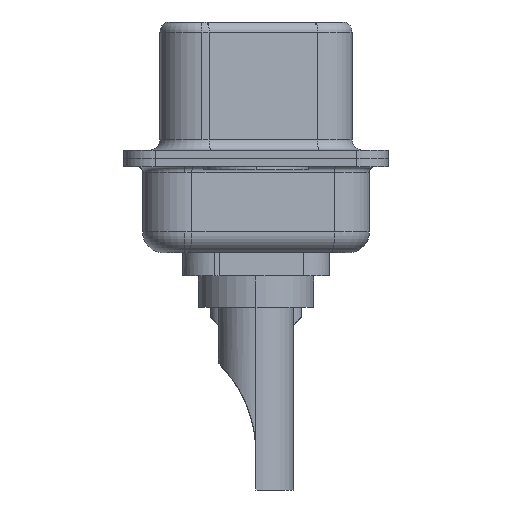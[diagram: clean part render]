
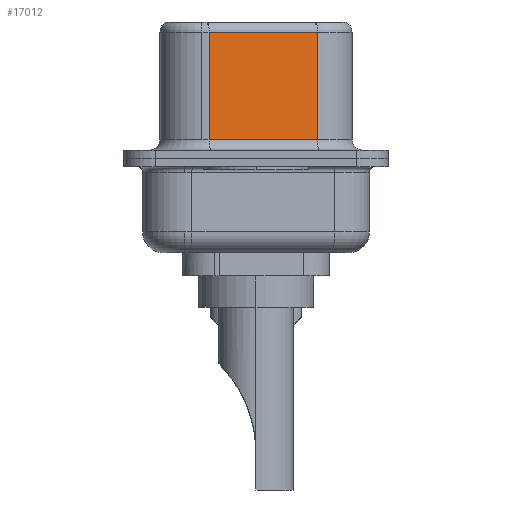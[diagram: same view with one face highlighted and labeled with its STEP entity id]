
A CAD part, left-side view. The second image highlights one B-rep face of the part: STEP entity #17012.
In plain terms, the highlighted planar face has unit normal (-0.985, -0.174, 0).
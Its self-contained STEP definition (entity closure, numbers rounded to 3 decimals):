
#373 = EDGE_CURVE ( 'NONE', #15705, #1648, #18455, .T. ) ;
#572 = CARTESIAN_POINT ( 'NONE',  ( 4.58, -2.927, 6.02 ) ) ;
#975 = VERTEX_POINT ( 'NONE', #13249 ) ;
#1648 = VERTEX_POINT ( 'NONE', #19920 ) ;
#2156 = CARTESIAN_POINT ( 'NONE',  ( 4.58, -2.927, 6.52 ) ) ;
#2408 = VECTOR ( 'NONE', #16342, 1000. ) ;
#2523 = ORIENTED_EDGE ( 'NONE', *, *, #3319, .T. ) ;
#3319 = EDGE_CURVE ( 'NONE', #15705, #975, #6019, .T. ) ;
#3413 = EDGE_CURVE ( 'NONE', #975, #19812, #15924, .T. ) ;
#3625 = VECTOR ( 'NONE', #8868, 1000. ) ;
#4381 = CARTESIAN_POINT ( 'NONE',  ( 4.58, -2.927, 0.9 ) ) ;
#6019 = LINE ( 'NONE', #572, #2408 ) ;
#6318 = DIRECTION ( 'NONE',  ( 0., 0., -1. ) ) ;
#6382 = FACE_OUTER_BOUND ( 'NONE', #16392, .T. ) ;
#6787 = DIRECTION ( 'NONE',  ( 0.985, 0.174, 0. ) ) ;
#7215 = EDGE_CURVE ( 'NONE', #19812, #1648, #11224, .T. ) ;
#7434 = CARTESIAN_POINT ( 'NONE',  ( 4.58, -2.927, 6.52 ) ) ;
#7708 = CARTESIAN_POINT ( 'NONE',  ( 4.58, -2.927, 6.02 ) ) ;
#8868 = DIRECTION ( 'NONE',  ( 0., 0., -1. ) ) ;
#10206 = ORIENTED_EDGE ( 'NONE', *, *, #3413, .T. ) ;
#10735 = VECTOR ( 'NONE', #18488, 1000. ) ;
#11224 = LINE ( 'NONE', #4381, #10735 ) ;
#13249 = CARTESIAN_POINT ( 'NONE',  ( 3.67, 2.233, 6.02 ) ) ;
#13509 = CARTESIAN_POINT ( 'NONE',  ( 3.67, 2.233, 0.9 ) ) ;
#14355 = VECTOR ( 'NONE', #6318, 1000. ) ;
#14700 = ORIENTED_EDGE ( 'NONE', *, *, #7215, .T. ) ;
#15705 = VERTEX_POINT ( 'NONE', #7708 ) ;
#15924 = LINE ( 'NONE', #18308, #3625 ) ;
#16036 = PLANE ( 'NONE',  #18332 ) ;
#16342 = DIRECTION ( 'NONE',  ( -0.174, 0.985, 0. ) ) ;
#16392 = EDGE_LOOP ( 'NONE', ( #19455, #2523, #10206, #14700 ) ) ;
#17012 = ADVANCED_FACE ( 'NONE', ( #6382 ), #16036, .F. ) ;
#17604 = DIRECTION ( 'NONE',  ( -0.174, 0.985, 0. ) ) ;
#18308 = CARTESIAN_POINT ( 'NONE',  ( 3.67, 2.233, 6.52 ) ) ;
#18332 = AXIS2_PLACEMENT_3D ( 'NONE', #2156, #6787, #17604 ) ;
#18455 = LINE ( 'NONE', #7434, #14355 ) ;
#18488 = DIRECTION ( 'NONE',  ( 0.174, -0.985, 0. ) ) ;
#19455 = ORIENTED_EDGE ( 'NONE', *, *, #373, .F. ) ;
#19812 = VERTEX_POINT ( 'NONE', #13509 ) ;
#19920 = CARTESIAN_POINT ( 'NONE',  ( 4.58, -2.927, 0.9 ) ) ;
